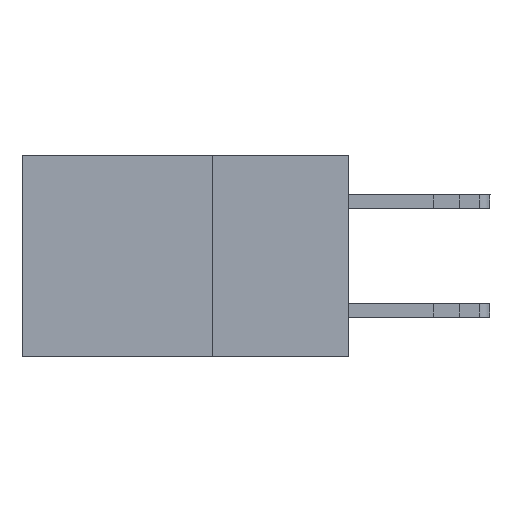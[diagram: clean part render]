
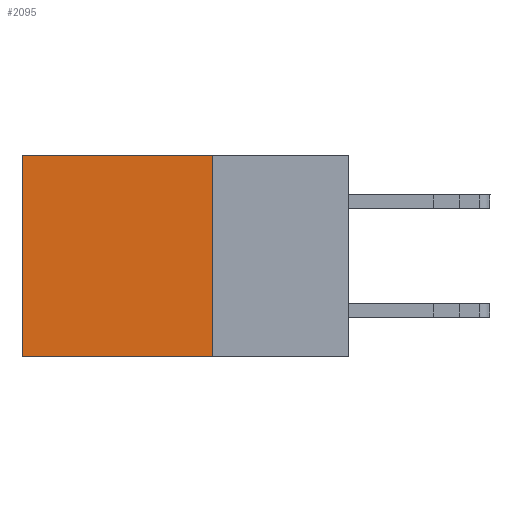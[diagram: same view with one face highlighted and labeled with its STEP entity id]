
A CAD part, left-side view. The second image highlights one B-rep face of the part: STEP entity #2095.
In plain terms, the highlighted planar face has unit normal (-1, 0, 0).
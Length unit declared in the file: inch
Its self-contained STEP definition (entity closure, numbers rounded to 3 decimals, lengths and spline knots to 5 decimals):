
#13 = VECTOR ( 'NONE', #16037, 39.37008 ) ;
#75 = CARTESIAN_POINT ( 'NONE',  ( 0.298, 0.25, -0.37 ) ) ;
#129 = VECTOR ( 'NONE', #16359, 39.37008 ) ;
#527 = CARTESIAN_POINT ( 'NONE',  ( 0.298, 0.6, 0. ) ) ;
#1120 = EDGE_CURVE ( 'NONE', #15276, #11658, #6329, .T. ) ;
#1703 = VECTOR ( 'NONE', #16258, 39.37008 ) ;
#2095 = ADVANCED_FACE ( 'NONE', ( #3330 ), #17416, .F. ) ;
#2810 = DIRECTION ( 'NONE',  ( 1., 0., 0. ) ) ;
#3330 = FACE_OUTER_BOUND ( 'NONE', #7853, .T. ) ;
#3337 = DIRECTION ( 'NONE',  ( 0., 0., -1. ) ) ;
#3528 = EDGE_CURVE ( 'NONE', #15276, #6384, #3990, .T. ) ;
#3990 = LINE ( 'NONE', #9315, #129 ) ;
#5218 = CARTESIAN_POINT ( 'NONE',  ( 0.298, 0.6, 0. ) ) ;
#6329 = LINE ( 'NONE', #22389, #20643 ) ;
#6384 = VERTEX_POINT ( 'NONE', #5218 ) ;
#7459 = LINE ( 'NONE', #527, #1703 ) ;
#7853 = EDGE_LOOP ( 'NONE', ( #11941, #9994, #12683, #12334 ) ) ;
#8027 = CARTESIAN_POINT ( 'NONE',  ( 0.298, 0.25, 0. ) ) ;
#8137 = DIRECTION ( 'NONE',  ( 0., 0., -1. ) ) ;
#8290 = VERTEX_POINT ( 'NONE', #9128 ) ;
#9128 = CARTESIAN_POINT ( 'NONE',  ( 0.298, 0.6, -0.37 ) ) ;
#9315 = CARTESIAN_POINT ( 'NONE',  ( 0.298, 0.25, 0. ) ) ;
#9994 = ORIENTED_EDGE ( 'NONE', *, *, #21358, .F. ) ;
#11658 = VERTEX_POINT ( 'NONE', #18693 ) ;
#11941 = ORIENTED_EDGE ( 'NONE', *, *, #16369, .T. ) ;
#12334 = ORIENTED_EDGE ( 'NONE', *, *, #3528, .T. ) ;
#12683 = ORIENTED_EDGE ( 'NONE', *, *, #1120, .F. ) ;
#15276 = VERTEX_POINT ( 'NONE', #8027 ) ;
#15602 = AXIS2_PLACEMENT_3D ( 'NONE', #18586, #2810, #8137 ) ;
#15927 = LINE ( 'NONE', #75, #13 ) ;
#16037 = DIRECTION ( 'NONE',  ( 0., 1., 0. ) ) ;
#16258 = DIRECTION ( 'NONE',  ( 0., 0., -1. ) ) ;
#16359 = DIRECTION ( 'NONE',  ( 0., 1., 0. ) ) ;
#16369 = EDGE_CURVE ( 'NONE', #6384, #8290, #7459, .T. ) ;
#17416 = PLANE ( 'NONE',  #15602 ) ;
#18586 = CARTESIAN_POINT ( 'NONE',  ( 0.298, 0.25, 0. ) ) ;
#18693 = CARTESIAN_POINT ( 'NONE',  ( 0.298, 0.25, -0.37 ) ) ;
#20643 = VECTOR ( 'NONE', #3337, 39.37008 ) ;
#21358 = EDGE_CURVE ( 'NONE', #11658, #8290, #15927, .T. ) ;
#22389 = CARTESIAN_POINT ( 'NONE',  ( 0.298, 0.25, 0. ) ) ;
